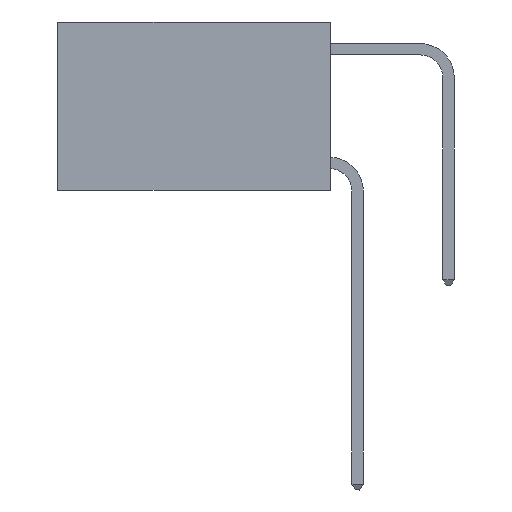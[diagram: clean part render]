
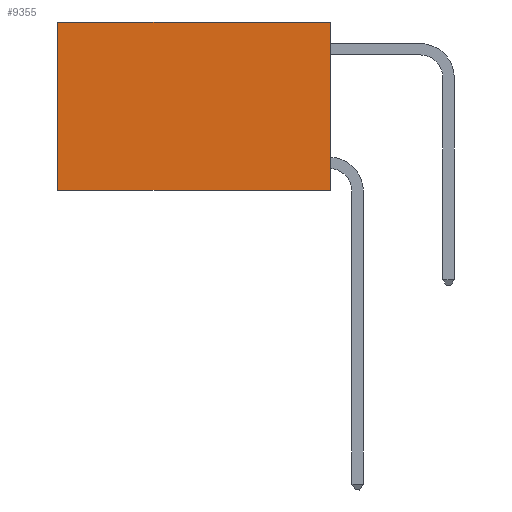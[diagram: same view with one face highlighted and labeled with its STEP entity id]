
A CAD part, left-side view. The second image highlights one B-rep face of the part: STEP entity #9355.
In plain terms, the highlighted planar face has unit normal (-1, 0, 0).
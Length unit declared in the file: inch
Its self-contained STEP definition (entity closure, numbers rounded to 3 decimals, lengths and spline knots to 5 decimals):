
#514 = VERTEX_POINT ( 'NONE', #13850 ) ;
#899 = EDGE_CURVE ( 'NONE', #8426, #514, #4824, .T. ) ;
#945 = VERTEX_POINT ( 'NONE', #12146 ) ;
#1261 = EDGE_CURVE ( 'NONE', #514, #4020, #9959, .T. ) ;
#3260 = EDGE_LOOP ( 'NONE', ( #14683, #5954, #15565, #6730 ) ) ;
#4020 = VERTEX_POINT ( 'NONE', #12041 ) ;
#4256 = VECTOR ( 'NONE', #11874, 39.37008 ) ;
#4824 = LINE ( 'NONE', #18870, #4256 ) ;
#4973 = CARTESIAN_POINT ( 'NONE',  ( 0.2625, 0.6, 0. ) ) ;
#5212 = AXIS2_PLACEMENT_3D ( 'NONE', #15651, #8597, #20896 ) ;
#5954 = ORIENTED_EDGE ( 'NONE', *, *, #1261, .F. ) ;
#6730 = ORIENTED_EDGE ( 'NONE', *, *, #19802, .T. ) ;
#8119 = CARTESIAN_POINT ( 'NONE',  ( 0.2625, 0., 0. ) ) ;
#8426 = VERTEX_POINT ( 'NONE', #8119 ) ;
#8597 = DIRECTION ( 'NONE',  ( 1., 0., 0. ) ) ;
#9162 = FACE_OUTER_BOUND ( 'NONE', #3260, .T. ) ;
#9355 = ADVANCED_FACE ( 'NONE', ( #9162 ), #19147, .F. ) ;
#9959 = LINE ( 'NONE', #20831, #13614 ) ;
#11874 = DIRECTION ( 'NONE',  ( 0., 0., -1. ) ) ;
#12041 = CARTESIAN_POINT ( 'NONE',  ( 0.2625, 0.6, -0.37 ) ) ;
#12146 = CARTESIAN_POINT ( 'NONE',  ( 0.2625, 0.6, 0. ) ) ;
#13614 = VECTOR ( 'NONE', #15394, 39.37008 ) ;
#13850 = CARTESIAN_POINT ( 'NONE',  ( 0.2625, 0., -0.37 ) ) ;
#14683 = ORIENTED_EDGE ( 'NONE', *, *, #18207, .T. ) ;
#15365 = CARTESIAN_POINT ( 'NONE',  ( 0.2625, 0., 0. ) ) ;
#15394 = DIRECTION ( 'NONE',  ( 0., 1., 0. ) ) ;
#15565 = ORIENTED_EDGE ( 'NONE', *, *, #899, .F. ) ;
#15651 = CARTESIAN_POINT ( 'NONE',  ( 0.2625, 0., 0. ) ) ;
#16668 = VECTOR ( 'NONE', #22485, 39.37008 ) ;
#16996 = VECTOR ( 'NONE', #17114, 39.37008 ) ;
#17114 = DIRECTION ( 'NONE',  ( 0., 1., 0. ) ) ;
#17547 = LINE ( 'NONE', #15365, #16996 ) ;
#18207 = EDGE_CURVE ( 'NONE', #945, #4020, #21295, .T. ) ;
#18870 = CARTESIAN_POINT ( 'NONE',  ( 0.2625, 0., 0. ) ) ;
#19147 = PLANE ( 'NONE',  #5212 ) ;
#19802 = EDGE_CURVE ( 'NONE', #8426, #945, #17547, .T. ) ;
#20831 = CARTESIAN_POINT ( 'NONE',  ( 0.2625, 0., -0.37 ) ) ;
#20896 = DIRECTION ( 'NONE',  ( 0., 0., -1. ) ) ;
#21295 = LINE ( 'NONE', #4973, #16668 ) ;
#22485 = DIRECTION ( 'NONE',  ( 0., 0., -1. ) ) ;
